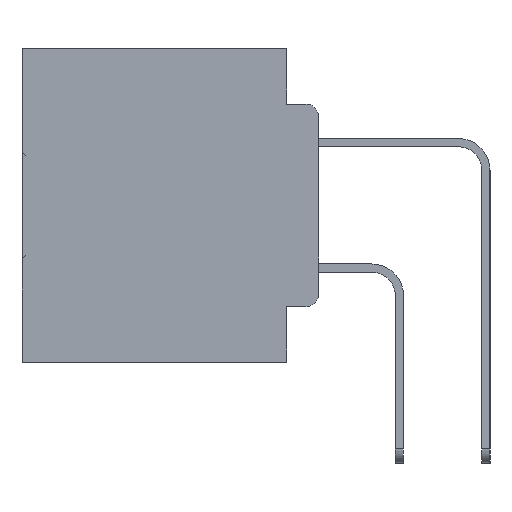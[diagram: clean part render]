
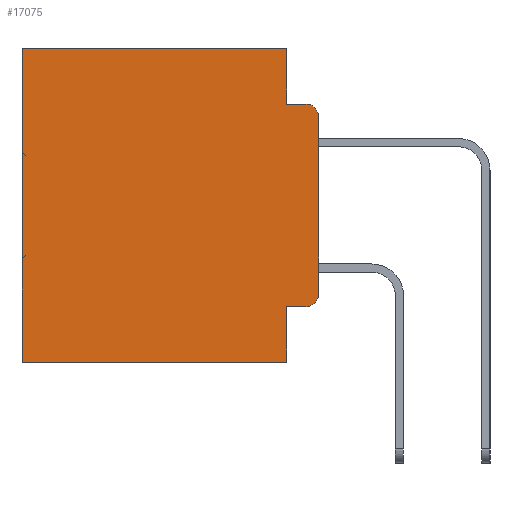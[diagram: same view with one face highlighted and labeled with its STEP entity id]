
A CAD part, left-side view. The second image highlights one B-rep face of the part: STEP entity #17075.
In plain terms, the highlighted planar face has unit normal (-1, 0, 0).
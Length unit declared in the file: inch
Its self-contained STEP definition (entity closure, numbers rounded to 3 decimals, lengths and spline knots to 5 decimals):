
#323 = EDGE_CURVE ( 'NONE', #23974, #3270, #15798, .T. ) ;
#1189 = CARTESIAN_POINT ( 'NONE',  ( 0.298, 0., 0. ) ) ;
#1273 = VERTEX_POINT ( 'NONE', #22266 ) ;
#1932 = CIRCLE ( 'NONE', #24433, 0.02 ) ;
#2133 = AXIS2_PLACEMENT_3D ( 'NONE', #20418, #3394, #23303 ) ;
#2235 = VECTOR ( 'NONE', #23236, 39.37008 ) ;
#3270 = VERTEX_POINT ( 'NONE', #12697 ) ;
#3318 = CARTESIAN_POINT ( 'NONE',  ( 0.298, 0.473, 0. ) ) ;
#3394 = DIRECTION ( 'NONE',  ( -1., 0., 0. ) ) ;
#5046 = EDGE_CURVE ( 'NONE', #1273, #16367, #21182, .T. ) ;
#5271 = DIRECTION ( 'NONE',  ( 0., 1., 0. ) ) ;
#5411 = ORIENTED_EDGE ( 'NONE', *, *, #22472, .T. ) ;
#5470 = DIRECTION ( 'NONE',  ( -1., 0., 0. ) ) ;
#5892 = FACE_OUTER_BOUND ( 'NONE', #19869, .T. ) ;
#6210 = VERTEX_POINT ( 'NONE', #21351 ) ;
#7264 = EDGE_CURVE ( 'NONE', #9707, #23974, #20424, .T. ) ;
#7688 = EDGE_CURVE ( 'NONE', #16367, #28093, #28755, .T. ) ;
#8243 = VECTOR ( 'NONE', #5271, 39.37008 ) ;
#8705 = CARTESIAN_POINT ( 'NONE',  ( 0.298, 0.051, -0.5 ) ) ;
#9707 = VERTEX_POINT ( 'NONE', #35388 ) ;
#9843 = LINE ( 'NONE', #3318, #2235 ) ;
#10441 = CARTESIAN_POINT ( 'NONE',  ( 0.298, 0.473, 0. ) ) ;
#10631 = ORIENTED_EDGE ( 'NONE', *, *, #12661, .T. ) ;
#10978 = CARTESIAN_POINT ( 'NONE',  ( 0.298, 0.051, -0.0885 ) ) ;
#11226 = CARTESIAN_POINT ( 'NONE',  ( 0.298, 0., 0. ) ) ;
#11259 = ORIENTED_EDGE ( 'NONE', *, *, #7688, .F. ) ;
#11371 = CARTESIAN_POINT ( 'NONE',  ( 0.298, 0.051, -0.0885 ) ) ;
#11740 = VERTEX_POINT ( 'NONE', #24959 ) ;
#11922 = ORIENTED_EDGE ( 'NONE', *, *, #7264, .F. ) ;
#12025 = ORIENTED_EDGE ( 'NONE', *, *, #5046, .F. ) ;
#12661 = EDGE_CURVE ( 'NONE', #11740, #28093, #21434, .T. ) ;
#12697 = CARTESIAN_POINT ( 'NONE',  ( 0.298, 0.473, -0.5 ) ) ;
#12749 = ORIENTED_EDGE ( 'NONE', *, *, #35995, .T. ) ;
#13058 = ORIENTED_EDGE ( 'NONE', *, *, #31830, .T. ) ;
#13322 = ORIENTED_EDGE ( 'NONE', *, *, #27166, .T. ) ;
#13665 = VECTOR ( 'NONE', #29205, 39.37008 ) ;
#14356 = DIRECTION ( 'NONE',  ( 0., -1., 0. ) ) ;
#14539 = VECTOR ( 'NONE', #14356, 39.37008 ) ;
#14602 = LINE ( 'NONE', #1189, #35261 ) ;
#14935 = DIRECTION ( 'NONE',  ( 0., 0., -1. ) ) ;
#14968 = CARTESIAN_POINT ( 'NONE',  ( 0.298, 0.051, 0. ) ) ;
#15776 = VECTOR ( 'NONE', #28126, 39.37008 ) ;
#15798 = LINE ( 'NONE', #18012, #8243 ) ;
#16367 = VERTEX_POINT ( 'NONE', #11371 ) ;
#17060 = CARTESIAN_POINT ( 'NONE',  ( 0.298, 0.051, -0.4115 ) ) ;
#17075 = ADVANCED_FACE ( 'NONE', ( #5892 ), #26203, .F. ) ;
#18012 = CARTESIAN_POINT ( 'NONE',  ( 0.298, 0., -0.5 ) ) ;
#19869 = EDGE_LOOP ( 'NONE', ( #35115, #10631, #11259, #12025, #12749, #13322, #22126, #11922, #5411, #13058 ) ) ;
#20418 = CARTESIAN_POINT ( 'NONE',  ( 0.298, 0.02, -0.1085 ) ) ;
#20424 = LINE ( 'NONE', #14968, #27925 ) ;
#20493 = CARTESIAN_POINT ( 'NONE',  ( 0.298, 0., 0. ) ) ;
#20708 = VERTEX_POINT ( 'NONE', #28742 ) ;
#21182 = LINE ( 'NONE', #34702, #13665 ) ;
#21351 = CARTESIAN_POINT ( 'NONE',  ( 0.298, 0., -0.3915 ) ) ;
#21434 = CIRCLE ( 'NONE', #2133, 0.02 ) ;
#21605 = EDGE_CURVE ( 'NONE', #11740, #6210, #14602, .T. ) ;
#22126 = ORIENTED_EDGE ( 'NONE', *, *, #323, .F. ) ;
#22266 = CARTESIAN_POINT ( 'NONE',  ( 0.298, 0.051, 0. ) ) ;
#22472 = EDGE_CURVE ( 'NONE', #9707, #20708, #29522, .T. ) ;
#22503 = CARTESIAN_POINT ( 'NONE',  ( 0.298, 0.02, -0.3915 ) ) ;
#23236 = DIRECTION ( 'NONE',  ( 0., 0., -1. ) ) ;
#23303 = DIRECTION ( 'NONE',  ( 0., 0., -1. ) ) ;
#23974 = VERTEX_POINT ( 'NONE', #8705 ) ;
#24433 = AXIS2_PLACEMENT_3D ( 'NONE', #22503, #5470, #25338 ) ;
#24959 = CARTESIAN_POINT ( 'NONE',  ( 0.298, 0., -0.1085 ) ) ;
#25338 = DIRECTION ( 'NONE',  ( 0., 0., -1. ) ) ;
#26203 = PLANE ( 'NONE',  #31384 ) ;
#26778 = DIRECTION ( 'NONE',  ( 0., 0., -1. ) ) ;
#27166 = EDGE_CURVE ( 'NONE', #36435, #3270, #9843, .T. ) ;
#27895 = DIRECTION ( 'NONE',  ( 0., -1., 0. ) ) ;
#27925 = VECTOR ( 'NONE', #31810, 39.37008 ) ;
#28093 = VERTEX_POINT ( 'NONE', #35838 ) ;
#28126 = DIRECTION ( 'NONE',  ( 0., 1., 0. ) ) ;
#28742 = CARTESIAN_POINT ( 'NONE',  ( 0.298, 0.02, -0.4115 ) ) ;
#28755 = LINE ( 'NONE', #10978, #35309 ) ;
#29205 = DIRECTION ( 'NONE',  ( 0., 0., -1. ) ) ;
#29522 = LINE ( 'NONE', #17060, #14539 ) ;
#31384 = AXIS2_PLACEMENT_3D ( 'NONE', #20493, #31777, #14935 ) ;
#31595 = LINE ( 'NONE', #11226, #15776 ) ;
#31777 = DIRECTION ( 'NONE',  ( 1., 0., 0. ) ) ;
#31810 = DIRECTION ( 'NONE',  ( 0., 0., -1. ) ) ;
#31830 = EDGE_CURVE ( 'NONE', #20708, #6210, #1932, .T. ) ;
#34702 = CARTESIAN_POINT ( 'NONE',  ( 0.298, 0.051, 0. ) ) ;
#35115 = ORIENTED_EDGE ( 'NONE', *, *, #21605, .F. ) ;
#35261 = VECTOR ( 'NONE', #26778, 39.37008 ) ;
#35309 = VECTOR ( 'NONE', #27895, 39.37008 ) ;
#35388 = CARTESIAN_POINT ( 'NONE',  ( 0.298, 0.051, -0.4115 ) ) ;
#35838 = CARTESIAN_POINT ( 'NONE',  ( 0.298, 0.02, -0.0885 ) ) ;
#35995 = EDGE_CURVE ( 'NONE', #1273, #36435, #31595, .T. ) ;
#36435 = VERTEX_POINT ( 'NONE', #10441 ) ;
